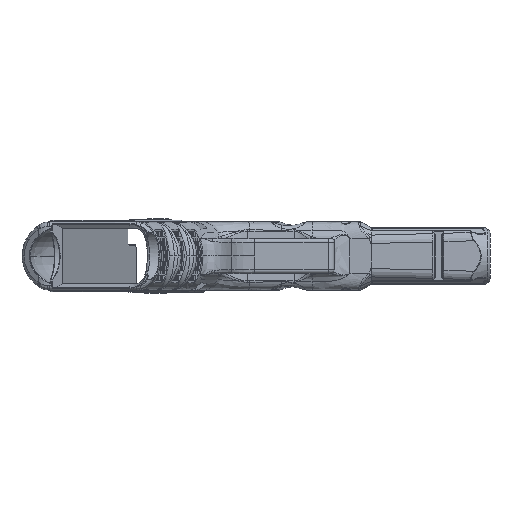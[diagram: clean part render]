
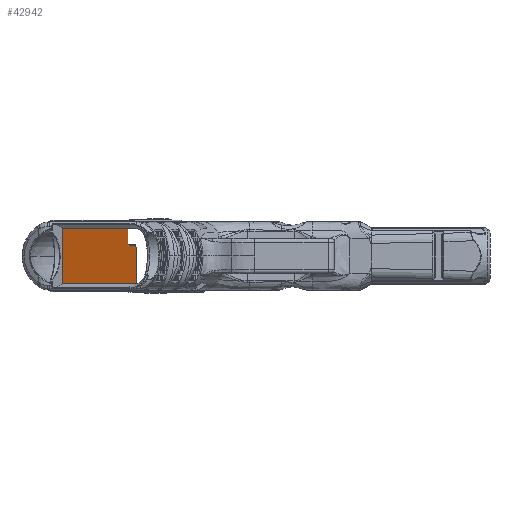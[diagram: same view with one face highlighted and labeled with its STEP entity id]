
A CAD part, front view. The second image highlights one B-rep face of the part: STEP entity #42942.
In plain terms, the highlighted planar face has unit normal (0.951, -0.309, 0).
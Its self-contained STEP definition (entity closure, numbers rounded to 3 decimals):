
#1502=LINE('',#61135,#4218);
#1903=LINE('',#71763,#4619);
#1904=LINE('',#71805,#4620);
#1905=LINE('',#71808,#4621);
#1906=LINE('',#71810,#4622);
#1907=LINE('',#71811,#4623);
#4218=VECTOR('',#49232,10.);
#4619=VECTOR('',#50635,10.);
#4620=VECTOR('',#50644,10.);
#4621=VECTOR('',#50647,1000.);
#4622=VECTOR('',#50648,10.);
#4623=VECTOR('',#50649,1000.);
#7013=PLANE('',#45761);
#7876=ELLIPSE('',#45759,0.536,0.51);
#9425=FACE_OUTER_BOUND('',#12010,.T.);
#12010=EDGE_LOOP('',(#29791,#29792,#29793,#29794,#29795,#29796,#29797));
#16949=VERTEX_POINT('',#61128);
#16952=VERTEX_POINT('',#61133);
#17627=VERTEX_POINT('',#71760);
#17628=VERTEX_POINT('',#71762);
#17629=VERTEX_POINT('',#71801);
#17630=VERTEX_POINT('',#71807);
#17631=VERTEX_POINT('',#71809);
#21374=EDGE_CURVE('',#16952,#16949,#1502,.T.);
#22286=EDGE_CURVE('',#17627,#17628,#1903,.T.);
#22289=EDGE_CURVE('',#17629,#17627,#7876,.T.);
#22290=EDGE_CURVE('',#16949,#17629,#1904,.T.);
#22291=EDGE_CURVE('',#17630,#16952,#1905,.T.);
#22292=EDGE_CURVE('',#17631,#17630,#1906,.T.);
#22293=EDGE_CURVE('',#17628,#17631,#1907,.T.);
#29791=ORIENTED_EDGE('',*,*,#21374,.F.);
#29792=ORIENTED_EDGE('',*,*,#22291,.F.);
#29793=ORIENTED_EDGE('',*,*,#22292,.F.);
#29794=ORIENTED_EDGE('',*,*,#22293,.F.);
#29795=ORIENTED_EDGE('',*,*,#22286,.F.);
#29796=ORIENTED_EDGE('',*,*,#22289,.F.);
#29797=ORIENTED_EDGE('',*,*,#22290,.F.);
#42942=ADVANCED_FACE('',(#9425),#7013,.F.);
#45759=AXIS2_PLACEMENT_3D('',#71803,#50640,#50641);
#45761=AXIS2_PLACEMENT_3D('',#71806,#50645,#50646);
#49232=DIRECTION('',(0.,0.,-1.));
#50635=DIRECTION('',(0.,0.,-1.));
#50640=DIRECTION('center_axis',(-0.951,0.309,0.));
#50641=DIRECTION('ref_axis',(0.309,0.951,0.));
#50644=DIRECTION('',(0.309,0.951,0.));
#50645=DIRECTION('center_axis',(-0.951,0.309,0.));
#50646=DIRECTION('ref_axis',(0.,0.,1.));
#50647=DIRECTION('',(0.309,0.951,0.));
#50648=DIRECTION('',(0.,0.,1.));
#50649=DIRECTION('',(-0.309,-0.951,0.));
#61128=CARTESIAN_POINT('',(29.972,-12.638,4.26));
#61133=CARTESIAN_POINT('',(29.972,-12.638,11.75));
#61135=CARTESIAN_POINT('',(29.972,-12.638,2.982));
#71760=CARTESIAN_POINT('',(33.382,-2.141,3.75));
#71762=CARTESIAN_POINT('',(33.382,-2.141,-11.75));
#71763=CARTESIAN_POINT('',(33.382,-2.141,-5.651));
#71801=CARTESIAN_POINT('',(33.216,-2.651,4.26));
#71803=CARTESIAN_POINT('Origin',(33.216,-2.651,3.75));
#71805=CARTESIAN_POINT('',(34.619,1.664,4.26));
#71806=CARTESIAN_POINT('Origin',(33.829,-0.765,-11.75));
#71807=CARTESIAN_POINT('',(2.236,-98.,11.75));
#71808=CARTESIAN_POINT('',(30.125,-12.165,11.75));
#71809=CARTESIAN_POINT('',(2.236,-98.,-11.75));
#71810=CARTESIAN_POINT('',(2.236,-98.,-18.375));
#71811=CARTESIAN_POINT('',(33.829,-0.765,-11.75));
